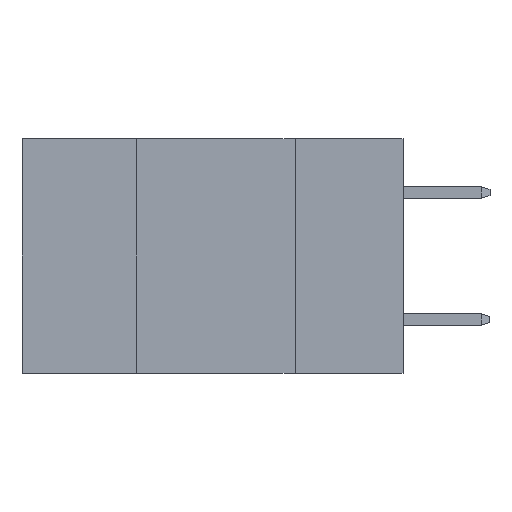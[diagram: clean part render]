
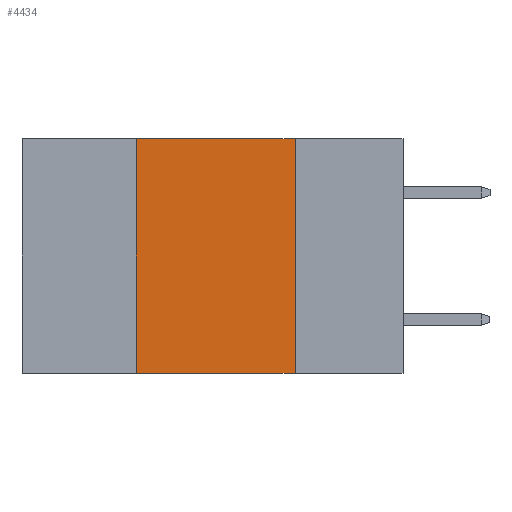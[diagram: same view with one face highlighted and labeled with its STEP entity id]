
A CAD part, left-side view. The second image highlights one B-rep face of the part: STEP entity #4434.
In plain terms, the highlighted planar face has unit normal (-1, 0, 0).
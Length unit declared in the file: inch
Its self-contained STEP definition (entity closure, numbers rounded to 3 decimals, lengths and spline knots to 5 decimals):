
#594 = VECTOR ( 'NONE', #7513, 39.37008 ) ;
#652 = ORIENTED_EDGE ( 'NONE', *, *, #9552, .F. ) ;
#974 = LINE ( 'NONE', #6815, #594 ) ;
#1133 = EDGE_CURVE ( 'NONE', #1884, #6246, #974, .T. ) ;
#1442 = VECTOR ( 'NONE', #4735, 39.37008 ) ;
#1632 = EDGE_CURVE ( 'NONE', #4435, #6001, #8869, .T. ) ;
#1884 = VERTEX_POINT ( 'NONE', #3226 ) ;
#1997 = CARTESIAN_POINT ( 'NONE',  ( 0., 0.17, -0.37 ) ) ;
#2032 = EDGE_LOOP ( 'NONE', ( #652, #8948, #3802, #5379 ) ) ;
#2434 = CARTESIAN_POINT ( 'NONE',  ( 0., 0.6, -0.37 ) ) ;
#2877 = VECTOR ( 'NONE', #3506, 39.37008 ) ;
#2969 = CARTESIAN_POINT ( 'NONE',  ( 0., 0.17, 0. ) ) ;
#3226 = CARTESIAN_POINT ( 'NONE',  ( 0., 0.42, 0. ) ) ;
#3253 = CARTESIAN_POINT ( 'NONE',  ( 0., 0.6, 0. ) ) ;
#3315 = CARTESIAN_POINT ( 'NONE',  ( 0., 0.42, -0.37 ) ) ;
#3420 = FACE_OUTER_BOUND ( 'NONE', #2032, .T. ) ;
#3506 = DIRECTION ( 'NONE',  ( 0., 0., 1. ) ) ;
#3802 = ORIENTED_EDGE ( 'NONE', *, *, #6943, .F. ) ;
#4434 = ADVANCED_FACE ( 'NONE', ( #3420 ), #9751, .F. ) ;
#4435 = VERTEX_POINT ( 'NONE', #3315 ) ;
#4735 = DIRECTION ( 'NONE',  ( 0., -1., 0. ) ) ;
#4966 = DIRECTION ( 'NONE',  ( 0., 0., -1. ) ) ;
#5323 = CARTESIAN_POINT ( 'NONE',  ( 0., 0.42, 0. ) ) ;
#5379 = ORIENTED_EDGE ( 'NONE', *, *, #1632, .T. ) ;
#6001 = VERTEX_POINT ( 'NONE', #1997 ) ;
#6246 = VERTEX_POINT ( 'NONE', #9774 ) ;
#6416 = DIRECTION ( 'NONE',  ( 1., 0., 0. ) ) ;
#6815 = CARTESIAN_POINT ( 'NONE',  ( 0., 0.6, 0. ) ) ;
#6943 = EDGE_CURVE ( 'NONE', #4435, #1884, #7735, .T. ) ;
#7513 = DIRECTION ( 'NONE',  ( 0., -1., 0. ) ) ;
#7735 = LINE ( 'NONE', #5323, #2877 ) ;
#7990 = LINE ( 'NONE', #2969, #8475 ) ;
#8475 = VECTOR ( 'NONE', #9413, 39.37008 ) ;
#8869 = LINE ( 'NONE', #2434, #1442 ) ;
#8948 = ORIENTED_EDGE ( 'NONE', *, *, #1133, .F. ) ;
#9413 = DIRECTION ( 'NONE',  ( 0., 0., -1. ) ) ;
#9552 = EDGE_CURVE ( 'NONE', #6246, #6001, #7990, .T. ) ;
#9565 = AXIS2_PLACEMENT_3D ( 'NONE', #3253, #6416, #4966 ) ;
#9751 = PLANE ( 'NONE',  #9565 ) ;
#9774 = CARTESIAN_POINT ( 'NONE',  ( 0., 0.17, 0. ) ) ;
